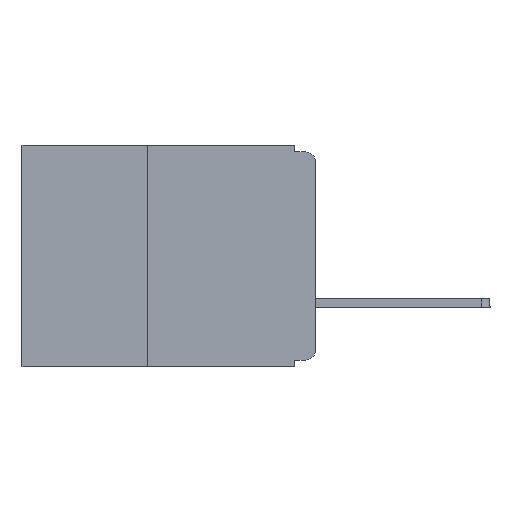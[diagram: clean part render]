
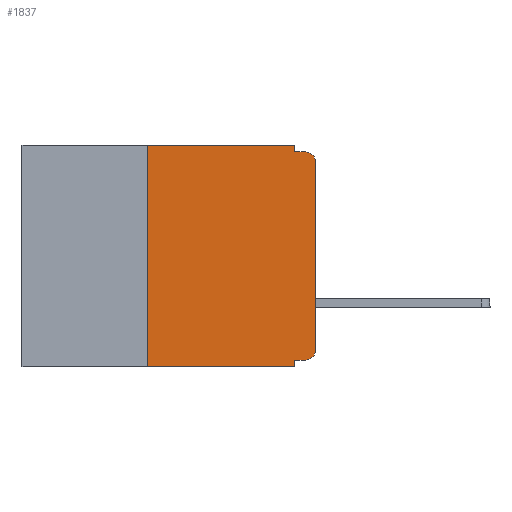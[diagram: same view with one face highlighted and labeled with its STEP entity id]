
A CAD part, left-side view. The second image highlights one B-rep face of the part: STEP entity #1837.
In plain terms, the highlighted planar face has unit normal (-1, 0, 0).
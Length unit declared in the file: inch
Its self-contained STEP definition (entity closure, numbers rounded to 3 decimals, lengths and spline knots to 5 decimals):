
#177 = CARTESIAN_POINT ( 'NONE',  ( 0., 0.015, -0.01 ) ) ;
#405 = CARTESIAN_POINT ( 'NONE',  ( 0., 0., -0.32 ) ) ;
#509 = DIRECTION ( 'NONE',  ( 0., 1., 0. ) ) ;
#609 = VERTEX_POINT ( 'NONE', #17348 ) ;
#1009 = DIRECTION ( 'NONE',  ( 0., -1., 0. ) ) ;
#1727 = EDGE_CURVE ( 'NONE', #9494, #26563, #9974, .T. ) ;
#1837 = ADVANCED_FACE ( 'NONE', ( #7065 ), #22807, .F. ) ;
#1930 = DIRECTION ( 'NONE',  ( 0., -1., 0. ) ) ;
#2041 = CARTESIAN_POINT ( 'NONE',  ( 0., 0.031, -0.01 ) ) ;
#2406 = LINE ( 'NONE', #14107, #13262 ) ;
#3031 = EDGE_CURVE ( 'NONE', #11687, #18400, #3728, .T. ) ;
#3315 = VERTEX_POINT ( 'NONE', #10450 ) ;
#3335 = LINE ( 'NONE', #26514, #21734 ) ;
#3728 = LINE ( 'NONE', #405, #28826 ) ;
#3820 = VECTOR ( 'NONE', #25255, 39.37008 ) ;
#3986 = VECTOR ( 'NONE', #24663, 39.37008 ) ;
#4549 = DIRECTION ( 'NONE',  ( -1., 0., 0. ) ) ;
#5170 = ORIENTED_EDGE ( 'NONE', *, *, #14746, .F. ) ;
#5391 = ORIENTED_EDGE ( 'NONE', *, *, #13480, .F. ) ;
#5490 = VECTOR ( 'NONE', #13214, 39.37008 ) ;
#6372 = EDGE_CURVE ( 'NONE', #7217, #22746, #23870, .T. ) ;
#6712 = VERTEX_POINT ( 'NONE', #23632 ) ;
#6818 = AXIS2_PLACEMENT_3D ( 'NONE', #23236, #22777, #22701 ) ;
#7065 = FACE_OUTER_BOUND ( 'NONE', #15008, .T. ) ;
#7217 = VERTEX_POINT ( 'NONE', #20794 ) ;
#7382 = ORIENTED_EDGE ( 'NONE', *, *, #18987, .T. ) ;
#8052 = CARTESIAN_POINT ( 'NONE',  ( 0., 0.015, -0.32 ) ) ;
#8724 = ORIENTED_EDGE ( 'NONE', *, *, #6372, .T. ) ;
#9125 = ORIENTED_EDGE ( 'NONE', *, *, #20073, .F. ) ;
#9188 = EDGE_CURVE ( 'NONE', #609, #3315, #11840, .T. ) ;
#9216 = ORIENTED_EDGE ( 'NONE', *, *, #1727, .F. ) ;
#9433 = CARTESIAN_POINT ( 'NONE',  ( 0., 0.015, -0.305 ) ) ;
#9494 = VERTEX_POINT ( 'NONE', #26038 ) ;
#9667 = CARTESIAN_POINT ( 'NONE',  ( 0., 0.031, -0.32 ) ) ;
#9974 = LINE ( 'NONE', #25472, #3820 ) ;
#10350 = CARTESIAN_POINT ( 'NONE',  ( 0., 0.437, 0. ) ) ;
#10450 = CARTESIAN_POINT ( 'NONE',  ( 0., 0.031, -0.33 ) ) ;
#11296 = EDGE_CURVE ( 'NONE', #22746, #14374, #20377, .T. ) ;
#11687 = VERTEX_POINT ( 'NONE', #8052 ) ;
#11766 = DIRECTION ( 'NONE',  ( 0., 0., -1. ) ) ;
#11840 = LINE ( 'NONE', #13462, #22607 ) ;
#12814 = DIRECTION ( 'NONE',  ( 0., 0., -1. ) ) ;
#13214 = DIRECTION ( 'NONE',  ( 0., 0., 1. ) ) ;
#13262 = VECTOR ( 'NONE', #21158, 39.37008 ) ;
#13462 = CARTESIAN_POINT ( 'NONE',  ( 0., 0.437, -0.33 ) ) ;
#13480 = EDGE_CURVE ( 'NONE', #18400, #3315, #3335, .T. ) ;
#14107 = CARTESIAN_POINT ( 'NONE',  ( 0., 0., -0.01 ) ) ;
#14374 = VERTEX_POINT ( 'NONE', #177 ) ;
#14629 = LINE ( 'NONE', #10350, #20028 ) ;
#14746 = EDGE_CURVE ( 'NONE', #609, #6712, #16263, .T. ) ;
#15008 = EDGE_LOOP ( 'NONE', ( #8724, #29231, #9125, #9216, #28644, #5170, #17276, #5391, #19426, #7382 ) ) ;
#16263 = LINE ( 'NONE', #20060, #3986 ) ;
#17276 = ORIENTED_EDGE ( 'NONE', *, *, #9188, .T. ) ;
#17348 = CARTESIAN_POINT ( 'NONE',  ( 0., 0.25, -0.33 ) ) ;
#18331 = CARTESIAN_POINT ( 'NONE',  ( 0., 0.015, -0.025 ) ) ;
#18400 = VERTEX_POINT ( 'NONE', #9667 ) ;
#18987 = EDGE_CURVE ( 'NONE', #11687, #7217, #27291, .T. ) ;
#19426 = ORIENTED_EDGE ( 'NONE', *, *, #3031, .F. ) ;
#19759 = AXIS2_PLACEMENT_3D ( 'NONE', #18331, #4549, #20642 ) ;
#20028 = VECTOR ( 'NONE', #1009, 39.37008 ) ;
#20035 = CARTESIAN_POINT ( 'NONE',  ( 0., 0., 0. ) ) ;
#20060 = CARTESIAN_POINT ( 'NONE',  ( 0., 0.25, -0.33 ) ) ;
#20073 = EDGE_CURVE ( 'NONE', #26563, #14374, #2406, .T. ) ;
#20377 = CIRCLE ( 'NONE', #19759, 0.015 ) ;
#20642 = DIRECTION ( 'NONE',  ( 0., 0., -1. ) ) ;
#20794 = CARTESIAN_POINT ( 'NONE',  ( 0., 0., -0.305 ) ) ;
#20923 = EDGE_CURVE ( 'NONE', #6712, #9494, #14629, .T. ) ;
#21158 = DIRECTION ( 'NONE',  ( 0., -1., 0. ) ) ;
#21734 = VECTOR ( 'NONE', #12814, 39.37008 ) ;
#22607 = VECTOR ( 'NONE', #1930, 39.37008 ) ;
#22701 = DIRECTION ( 'NONE',  ( 0., 0., -1. ) ) ;
#22746 = VERTEX_POINT ( 'NONE', #23419 ) ;
#22777 = DIRECTION ( 'NONE',  ( 1., 0., 0. ) ) ;
#22807 = PLANE ( 'NONE',  #6818 ) ;
#23236 = CARTESIAN_POINT ( 'NONE',  ( 0., 0.437, 0. ) ) ;
#23419 = CARTESIAN_POINT ( 'NONE',  ( 0., 0., -0.025 ) ) ;
#23632 = CARTESIAN_POINT ( 'NONE',  ( 0., 0.25, 0. ) ) ;
#23870 = LINE ( 'NONE', #20035, #5490 ) ;
#24663 = DIRECTION ( 'NONE',  ( 0., 0., 1. ) ) ;
#25255 = DIRECTION ( 'NONE',  ( 0., 0., -1. ) ) ;
#25472 = CARTESIAN_POINT ( 'NONE',  ( 0., 0.031, 0. ) ) ;
#25480 = DIRECTION ( 'NONE',  ( -1., 0., 0. ) ) ;
#26038 = CARTESIAN_POINT ( 'NONE',  ( 0., 0.031, 0. ) ) ;
#26514 = CARTESIAN_POINT ( 'NONE',  ( 0., 0.031, -0.33 ) ) ;
#26563 = VERTEX_POINT ( 'NONE', #2041 ) ;
#26966 = AXIS2_PLACEMENT_3D ( 'NONE', #9433, #25480, #11766 ) ;
#27291 = CIRCLE ( 'NONE', #26966, 0.015 ) ;
#28644 = ORIENTED_EDGE ( 'NONE', *, *, #20923, .F. ) ;
#28826 = VECTOR ( 'NONE', #509, 39.37008 ) ;
#29231 = ORIENTED_EDGE ( 'NONE', *, *, #11296, .T. ) ;
